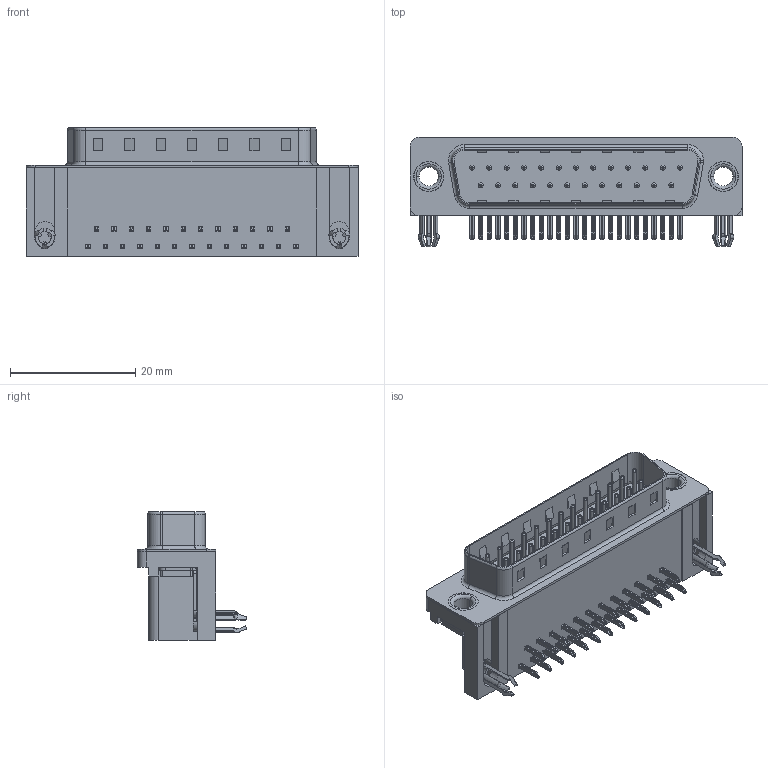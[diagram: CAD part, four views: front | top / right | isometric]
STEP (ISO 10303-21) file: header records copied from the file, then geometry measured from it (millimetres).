
FILE_DESCRIPTION (( 'STEP AP203' ), '1' );
FILE_NAME ('629-025-240-541.STEP', '2021-09-21T20:32:08', ( '' ), ( '' ), 'SwSTEP 2.0', 'SolidWorks 2020', '' );
FILE_SCHEMA (( 'CONFIG_CONTROL_DESIGN' ));
Length unit declared in the file: millimetre
Products named in the file (7): 629-025-240-541; 629 Housing_25 Socket; 629 Contact Bottom; 629 Thru Hole Rivet; 629 3 Prong Board Lock; 629 Shell_25 Socket; 629 Contact Top
Assembly tree (31 placements, depth 2):
  629-025-240-541
    629 Housing_25 Socket
    629 Shell_25 Socket
    629 Contact Bottom  x12
    629 Contact Top  x13
    629 3 Prong Board Lock  x2
    629 Thru Hole Rivet  x2
Bounding box: 53.04 x 17.48 x 20.6 mm (x, y, z)
Volume: 7323.5 mm3; surface area: 8283.1 mm2
Topology: 31 solids, 31 shells, 2325 faces, 5799 edges, 3593 vertices
Faces by surface type: plane 1441, cylinder 647, torus 201, cone 36
Entity records: 22051 total; most frequent: DIRECTION 3656, CARTESIAN_POINT 3582, ORIENTED_EDGE 3454, EDGE_CURVE 1727, AXIS2_PLACEMENT_3D 1221, VECTOR 1214, LINE 1214, VERTEX_POINT 1111
